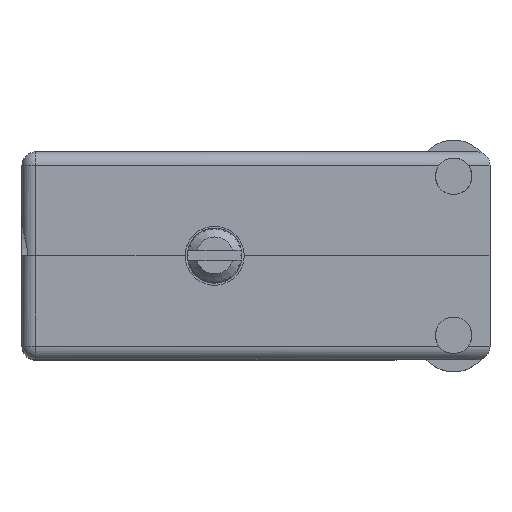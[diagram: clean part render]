
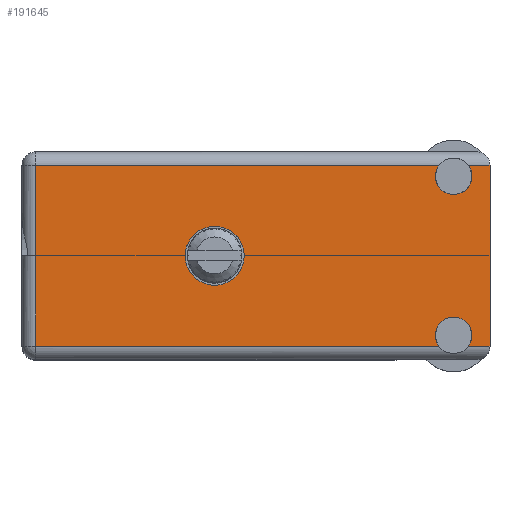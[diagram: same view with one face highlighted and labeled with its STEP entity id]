
A CAD part, top view. The second image highlights one B-rep face of the part: STEP entity #191645.
In plain terms, the highlighted face is planar.
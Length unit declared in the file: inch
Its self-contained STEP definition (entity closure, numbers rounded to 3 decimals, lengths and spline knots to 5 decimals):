
#2105 = DIRECTION ( 'NONE',  ( 0., 1., 0. ) ) ;
#2344 = ORIENTED_EDGE ( 'NONE', *, *, #168164, .F. ) ;
#3025 = EDGE_LOOP ( 'NONE', ( #114183, #20123, #40495, #165628, #141887, #57804, #52240, #194778, #90305, #139857 ) ) ;
#4445 = VECTOR ( 'NONE', #155249, 39.37008 ) ;
#6917 = DIRECTION ( 'NONE',  ( 1., 0., 0. ) ) ;
#8493 = LINE ( 'NONE', #23753, #87810 ) ;
#8963 = CARTESIAN_POINT ( 'NONE',  ( 0.8215, 0.806, -0.211 ) ) ;
#11049 = LINE ( 'NONE', #152376, #61664 ) ;
#11632 = CARTESIAN_POINT ( 'NONE',  ( 0., 0.806, -0.1015 ) ) ;
#12544 = VERTEX_POINT ( 'NONE', #64221 ) ;
#14094 = LINE ( 'NONE', #139766, #4445 ) ;
#18519 = EDGE_CURVE ( 'NONE', #172454, #161476, #11049, .T. ) ;
#18751 = LINE ( 'NONE', #113482, #122297 ) ;
#19386 = CARTESIAN_POINT ( 'NONE',  ( -0.6625, 0.806, -0.3575 ) ) ;
#19772 = CARTESIAN_POINT ( 'NONE',  ( -0.6155, 0.806, 0.3105 ) ) ;
#20123 = ORIENTED_EDGE ( 'NONE', *, *, #83074, .F. ) ;
#21218 = DIRECTION ( 'NONE',  ( 1., 0., 0. ) ) ;
#22669 = VECTOR ( 'NONE', #51431, 39.37008 ) ;
#23753 = CARTESIAN_POINT ( 'NONE',  ( -0.6625, 0.806, -0.3105 ) ) ;
#24759 = EDGE_CURVE ( 'NONE', #185185, #169335, #18751, .T. ) ;
#25805 = CARTESIAN_POINT ( 'NONE',  ( 0.9465, 0.806, -0.3105 ) ) ;
#26295 = CARTESIAN_POINT ( 'NONE',  ( 0.8215, 0.806, 0.211 ) ) ;
#26986 = AXIS2_PLACEMENT_3D ( 'NONE', #180110, #59589, #57614 ) ;
#27326 = FACE_BOUND ( 'NONE', #169473, .T. ) ;
#31163 = DIRECTION ( 'NONE',  ( 0., 0., 1. ) ) ;
#34839 = VERTEX_POINT ( 'NONE', #114679 ) ;
#34854 = PLANE ( 'NONE',  #170310 ) ;
#40495 = ORIENTED_EDGE ( 'NONE', *, *, #84137, .F. ) ;
#41430 = CIRCLE ( 'NONE', #74172, 0.0625 ) ;
#44125 = AXIS2_PLACEMENT_3D ( 'NONE', #47117, #153413, #154769 ) ;
#45938 = EDGE_CURVE ( 'NONE', #34839, #144216, #186800, .T. ) ;
#46262 = AXIS2_PLACEMENT_3D ( 'NONE', #128372, #50956, #63738 ) ;
#47117 = CARTESIAN_POINT ( 'NONE',  ( 0.8215, 0.806, 0.2735 ) ) ;
#47202 = VECTOR ( 'NONE', #6917, 39.37008 ) ;
#49348 = LINE ( 'NONE', #173938, #22669 ) ;
#50956 = DIRECTION ( 'NONE',  ( 0., 1., 0. ) ) ;
#51431 = DIRECTION ( 'NONE',  ( 0., 0., 1. ) ) ;
#51483 = FACE_OUTER_BOUND ( 'NONE', #3025, .T. ) ;
#52240 = ORIENTED_EDGE ( 'NONE', *, *, #122256, .F. ) ;
#55853 = VERTEX_POINT ( 'NONE', #26295 ) ;
#57614 = DIRECTION ( 'NONE',  ( 0., 0., 1. ) ) ;
#57804 = ORIENTED_EDGE ( 'NONE', *, *, #18519, .T. ) ;
#58482 = VERTEX_POINT ( 'NONE', #19772 ) ;
#59589 = DIRECTION ( 'NONE',  ( 0., 1., 0. ) ) ;
#61664 = VECTOR ( 'NONE', #120174, 39.37008 ) ;
#63738 = DIRECTION ( 'NONE',  ( 0., 0., 1. ) ) ;
#64221 = CARTESIAN_POINT ( 'NONE',  ( -0.6155, 0.806, -0.3105 ) ) ;
#72529 = VERTEX_POINT ( 'NONE', #11632 ) ;
#73999 = CARTESIAN_POINT ( 'NONE',  ( 0.77113, 0.806, 0.3105 ) ) ;
#74172 = AXIS2_PLACEMENT_3D ( 'NONE', #97979, #113544, #129024 ) ;
#79204 = EDGE_CURVE ( 'NONE', #12544, #58482, #14094, .T. ) ;
#83074 = EDGE_CURVE ( 'NONE', #55853, #181912, #165160, .T. ) ;
#84137 = EDGE_CURVE ( 'NONE', #185185, #55853, #104680, .T. ) ;
#86526 = EDGE_CURVE ( 'NONE', #172454, #169335, #49348, .T. ) ;
#86682 = CIRCLE ( 'NONE', #46262, 0.1015 ) ;
#87810 = VECTOR ( 'NONE', #177880, 39.37008 ) ;
#88055 = LINE ( 'NONE', #146917, #47202 ) ;
#90305 = ORIENTED_EDGE ( 'NONE', *, *, #186928, .T. ) ;
#97979 = CARTESIAN_POINT ( 'NONE',  ( 0.8215, 0.806, -0.2735 ) ) ;
#104680 = CIRCLE ( 'NONE', #44125, 0.0625 ) ;
#107613 = CARTESIAN_POINT ( 'NONE',  ( 0., 0.806, 0.1015 ) ) ;
#107818 = CARTESIAN_POINT ( 'NONE',  ( 0.87187, 0.806, 0.3105 ) ) ;
#111687 = CIRCLE ( 'NONE', #174121, 0.1015 ) ;
#112299 = DIRECTION ( 'NONE',  ( -1., 0., 0. ) ) ;
#113482 = CARTESIAN_POINT ( 'NONE',  ( 0.9465, 0.806, 0.3105 ) ) ;
#113544 = DIRECTION ( 'NONE',  ( 0., 1., 0. ) ) ;
#114183 = ORIENTED_EDGE ( 'NONE', *, *, #149073, .T. ) ;
#114679 = CARTESIAN_POINT ( 'NONE',  ( 0.77113, 0.806, -0.3105 ) ) ;
#120174 = DIRECTION ( 'NONE',  ( -1., 0., 0. ) ) ;
#122256 = EDGE_CURVE ( 'NONE', #144216, #161476, #41430, .T. ) ;
#122297 = VECTOR ( 'NONE', #21218, 39.37008 ) ;
#125828 = DIRECTION ( 'NONE',  ( 0., 1., 0. ) ) ;
#128372 = CARTESIAN_POINT ( 'NONE',  ( 0., 0.806, 0. ) ) ;
#129024 = DIRECTION ( 'NONE',  ( 0., 0., 1. ) ) ;
#135939 = AXIS2_PLACEMENT_3D ( 'NONE', #156287, #2105, #187259 ) ;
#139766 = CARTESIAN_POINT ( 'NONE',  ( -0.6155, 0.806, -0.3575 ) ) ;
#139857 = ORIENTED_EDGE ( 'NONE', *, *, #79204, .T. ) ;
#139921 = EDGE_CURVE ( 'NONE', #72529, #198805, #86682, .T. ) ;
#141887 = ORIENTED_EDGE ( 'NONE', *, *, #86526, .F. ) ;
#144216 = VERTEX_POINT ( 'NONE', #8963 ) ;
#146917 = CARTESIAN_POINT ( 'NONE',  ( 0.9465, 0.806, 0.3105 ) ) ;
#149073 = EDGE_CURVE ( 'NONE', #58482, #181912, #88055, .T. ) ;
#152376 = CARTESIAN_POINT ( 'NONE',  ( -0.6625, 0.806, -0.3105 ) ) ;
#153413 = DIRECTION ( 'NONE',  ( 0., 1., 0. ) ) ;
#154769 = DIRECTION ( 'NONE',  ( 0., 0., 1. ) ) ;
#155249 = DIRECTION ( 'NONE',  ( 0., 0., 1. ) ) ;
#156287 = CARTESIAN_POINT ( 'NONE',  ( 0.8215, 0.806, -0.2735 ) ) ;
#156327 = DIRECTION ( 'NONE',  ( 0., 1., 0. ) ) ;
#161476 = VERTEX_POINT ( 'NONE', #179853 ) ;
#164680 = CARTESIAN_POINT ( 'NONE',  ( 0.9465, 0.806, 0.3105 ) ) ;
#165160 = CIRCLE ( 'NONE', #26986, 0.0625 ) ;
#165628 = ORIENTED_EDGE ( 'NONE', *, *, #24759, .T. ) ;
#168164 = EDGE_CURVE ( 'NONE', #198805, #72529, #111687, .T. ) ;
#169170 = CARTESIAN_POINT ( 'NONE',  ( 0., 0.806, 0. ) ) ;
#169335 = VERTEX_POINT ( 'NONE', #164680 ) ;
#169473 = EDGE_LOOP ( 'NONE', ( #2344, #188245 ) ) ;
#170310 = AXIS2_PLACEMENT_3D ( 'NONE', #19386, #125828, #112299 ) ;
#172454 = VERTEX_POINT ( 'NONE', #25805 ) ;
#173938 = CARTESIAN_POINT ( 'NONE',  ( 0.9465, 0.806, 0.3575 ) ) ;
#174121 = AXIS2_PLACEMENT_3D ( 'NONE', #169170, #156327, #31163 ) ;
#177880 = DIRECTION ( 'NONE',  ( -1., 0., 0. ) ) ;
#179853 = CARTESIAN_POINT ( 'NONE',  ( 0.87187, 0.806, -0.3105 ) ) ;
#180110 = CARTESIAN_POINT ( 'NONE',  ( 0.8215, 0.806, 0.2735 ) ) ;
#181912 = VERTEX_POINT ( 'NONE', #73999 ) ;
#185185 = VERTEX_POINT ( 'NONE', #107818 ) ;
#186800 = CIRCLE ( 'NONE', #135939, 0.0625 ) ;
#186928 = EDGE_CURVE ( 'NONE', #34839, #12544, #8493, .T. ) ;
#187259 = DIRECTION ( 'NONE',  ( 0., 0., 1. ) ) ;
#188245 = ORIENTED_EDGE ( 'NONE', *, *, #139921, .F. ) ;
#191645 = ADVANCED_FACE ( 'NONE', ( #27326, #51483 ), #34854, .T. ) ;
#194778 = ORIENTED_EDGE ( 'NONE', *, *, #45938, .F. ) ;
#198805 = VERTEX_POINT ( 'NONE', #107613 ) ;
